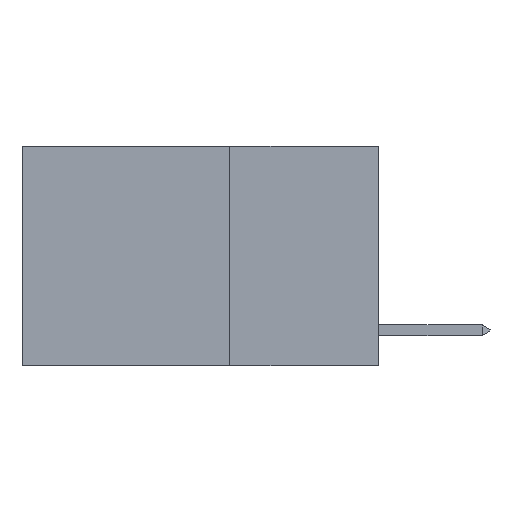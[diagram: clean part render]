
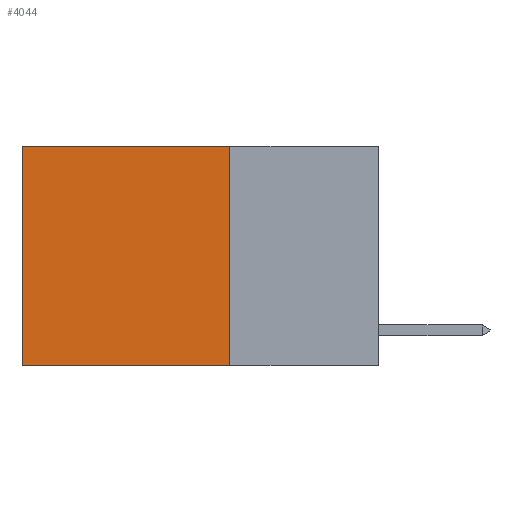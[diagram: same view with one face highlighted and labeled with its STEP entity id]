
A CAD part, left-side view. The second image highlights one B-rep face of the part: STEP entity #4044.
In plain terms, the highlighted planar face has unit normal (-1, 0, 0).
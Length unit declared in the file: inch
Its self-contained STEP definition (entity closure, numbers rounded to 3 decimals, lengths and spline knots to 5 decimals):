
#519 = LINE ( 'NONE', #14041, #19607 ) ;
#688 = VECTOR ( 'NONE', #19348, 39.37008 ) ;
#1413 = VECTOR ( 'NONE', #15759, 39.37008 ) ;
#1480 = CARTESIAN_POINT ( 'NONE',  ( 0.2625, 0.25, -0.37 ) ) ;
#1663 = EDGE_CURVE ( 'NONE', #5637, #23543, #519, .T. ) ;
#2705 = VECTOR ( 'NONE', #12772, 39.37008 ) ;
#4044 = ADVANCED_FACE ( 'NONE', ( #21829 ), #15667, .F. ) ;
#5637 = VERTEX_POINT ( 'NONE', #18591 ) ;
#6338 = AXIS2_PLACEMENT_3D ( 'NONE', #6405, #6489, #19347 ) ;
#6367 = LINE ( 'NONE', #8390, #1413 ) ;
#6405 = CARTESIAN_POINT ( 'NONE',  ( 0.2625, 0.25, 0. ) ) ;
#6489 = DIRECTION ( 'NONE',  ( 1., 0., 0. ) ) ;
#7012 = EDGE_CURVE ( 'NONE', #23543, #7451, #12565, .T. ) ;
#7451 = VERTEX_POINT ( 'NONE', #23203 ) ;
#7515 = ORIENTED_EDGE ( 'NONE', *, *, #1663, .T. ) ;
#7602 = VERTEX_POINT ( 'NONE', #1480 ) ;
#8390 = CARTESIAN_POINT ( 'NONE',  ( 0.2625, 0.25, -0.37 ) ) ;
#10613 = LINE ( 'NONE', #15668, #688 ) ;
#10955 = CARTESIAN_POINT ( 'NONE',  ( 0.2625, 0.6, 0. ) ) ;
#12565 = LINE ( 'NONE', #10955, #2705 ) ;
#12691 = ORIENTED_EDGE ( 'NONE', *, *, #7012, .T. ) ;
#12772 = DIRECTION ( 'NONE',  ( 0., 0., -1. ) ) ;
#14041 = CARTESIAN_POINT ( 'NONE',  ( 0.2625, 0.25, 0. ) ) ;
#15667 = PLANE ( 'NONE',  #6338 ) ;
#15668 = CARTESIAN_POINT ( 'NONE',  ( 0.2625, 0.25, 0. ) ) ;
#15759 = DIRECTION ( 'NONE',  ( 0., 1., 0. ) ) ;
#17328 = EDGE_CURVE ( 'NONE', #5637, #7602, #10613, .T. ) ;
#18416 = ORIENTED_EDGE ( 'NONE', *, *, #21083, .F. ) ;
#18591 = CARTESIAN_POINT ( 'NONE',  ( 0.2625, 0.25, 0. ) ) ;
#19347 = DIRECTION ( 'NONE',  ( 0., 0., -1. ) ) ;
#19348 = DIRECTION ( 'NONE',  ( 0., 0., -1. ) ) ;
#19372 = ORIENTED_EDGE ( 'NONE', *, *, #17328, .F. ) ;
#19607 = VECTOR ( 'NONE', #21460, 39.37008 ) ;
#21083 = EDGE_CURVE ( 'NONE', #7602, #7451, #6367, .T. ) ;
#21311 = CARTESIAN_POINT ( 'NONE',  ( 0.2625, 0.6, 0. ) ) ;
#21460 = DIRECTION ( 'NONE',  ( 0., 1., 0. ) ) ;
#21829 = FACE_OUTER_BOUND ( 'NONE', #22168, .T. ) ;
#22168 = EDGE_LOOP ( 'NONE', ( #12691, #18416, #19372, #7515 ) ) ;
#23203 = CARTESIAN_POINT ( 'NONE',  ( 0.2625, 0.6, -0.37 ) ) ;
#23543 = VERTEX_POINT ( 'NONE', #21311 ) ;
